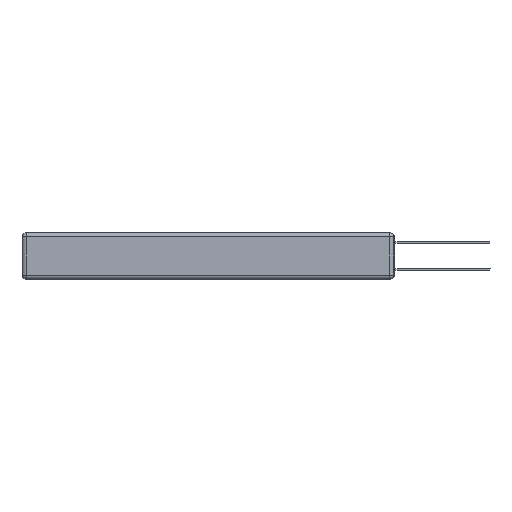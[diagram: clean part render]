
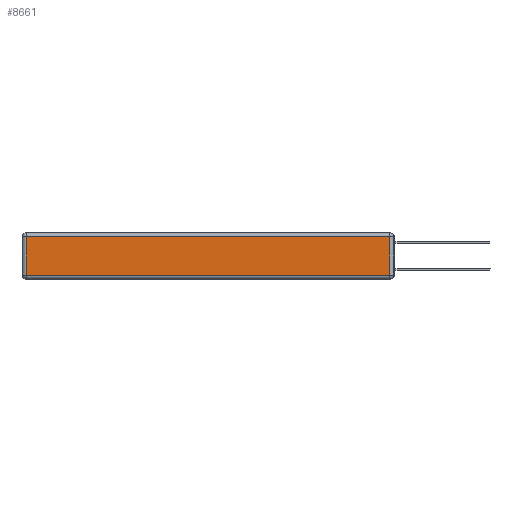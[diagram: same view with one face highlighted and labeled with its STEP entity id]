
A CAD part, left-side view. The second image highlights one B-rep face of the part: STEP entity #8661.
In plain terms, the highlighted planar face has unit normal (-1, 0, 0).
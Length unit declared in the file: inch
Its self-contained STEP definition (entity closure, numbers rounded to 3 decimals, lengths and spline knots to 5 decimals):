
#113 = VERTEX_POINT ( 'NONE', #11206 ) ;
#135 = LINE ( 'NONE', #1092, #8533 ) ;
#205 = VERTEX_POINT ( 'NONE', #4160 ) ;
#289 = VERTEX_POINT ( 'NONE', #12554 ) ;
#481 = CARTESIAN_POINT ( 'NONE',  ( 0., 2.72, -0.03 ) ) ;
#826 = CARTESIAN_POINT ( 'NONE',  ( 0., 0., -0.313 ) ) ;
#1092 = CARTESIAN_POINT ( 'NONE',  ( 0., 0.03, -0.343 ) ) ;
#2011 = VECTOR ( 'NONE', #3053, 39.37008 ) ;
#2696 = EDGE_LOOP ( 'NONE', ( #12194, #5858, #4929, #7281 ) ) ;
#2829 = LINE ( 'NONE', #13868, #2011 ) ;
#3053 = DIRECTION ( 'NONE',  ( 0., 0., -1. ) ) ;
#3383 = CARTESIAN_POINT ( 'NONE',  ( 0., 0., -0.343 ) ) ;
#3543 = DIRECTION ( 'NONE',  ( 0., 0., 1. ) ) ;
#3841 = LINE ( 'NONE', #7395, #6083 ) ;
#4160 = CARTESIAN_POINT ( 'NONE',  ( 0., 0.03, -0.313 ) ) ;
#4929 = ORIENTED_EDGE ( 'NONE', *, *, #12466, .T. ) ;
#5858 = ORIENTED_EDGE ( 'NONE', *, *, #8027, .T. ) ;
#6083 = VECTOR ( 'NONE', #12236, 39.37008 ) ;
#7086 = PLANE ( 'NONE',  #12844 ) ;
#7281 = ORIENTED_EDGE ( 'NONE', *, *, #10691, .T. ) ;
#7395 = CARTESIAN_POINT ( 'NONE',  ( 0., 2.75, -0.03 ) ) ;
#8027 = EDGE_CURVE ( 'NONE', #205, #289, #135, .T. ) ;
#8533 = VECTOR ( 'NONE', #9660, 39.37008 ) ;
#8661 = ADVANCED_FACE ( 'NONE', ( #11841 ), #7086, .T. ) ;
#9660 = DIRECTION ( 'NONE',  ( 0., 0., 1. ) ) ;
#10423 = DIRECTION ( 'NONE',  ( 0., -1., 0. ) ) ;
#10691 = EDGE_CURVE ( 'NONE', #12628, #113, #2829, .T. ) ;
#10842 = VECTOR ( 'NONE', #10423, 39.37008 ) ;
#11206 = CARTESIAN_POINT ( 'NONE',  ( 0., 2.72, -0.313 ) ) ;
#11248 = EDGE_CURVE ( 'NONE', #113, #205, #12905, .T. ) ;
#11841 = FACE_OUTER_BOUND ( 'NONE', #2696, .T. ) ;
#12194 = ORIENTED_EDGE ( 'NONE', *, *, #11248, .T. ) ;
#12236 = DIRECTION ( 'NONE',  ( 0., 1., 0. ) ) ;
#12466 = EDGE_CURVE ( 'NONE', #289, #12628, #3841, .T. ) ;
#12554 = CARTESIAN_POINT ( 'NONE',  ( 0., 0.03, -0.03 ) ) ;
#12628 = VERTEX_POINT ( 'NONE', #481 ) ;
#12844 = AXIS2_PLACEMENT_3D ( 'NONE', #3383, #13032, #3543 ) ;
#12905 = LINE ( 'NONE', #826, #10842 ) ;
#13032 = DIRECTION ( 'NONE',  ( -1., 0., 0. ) ) ;
#13868 = CARTESIAN_POINT ( 'NONE',  ( 0., 2.72, -0.343 ) ) ;
